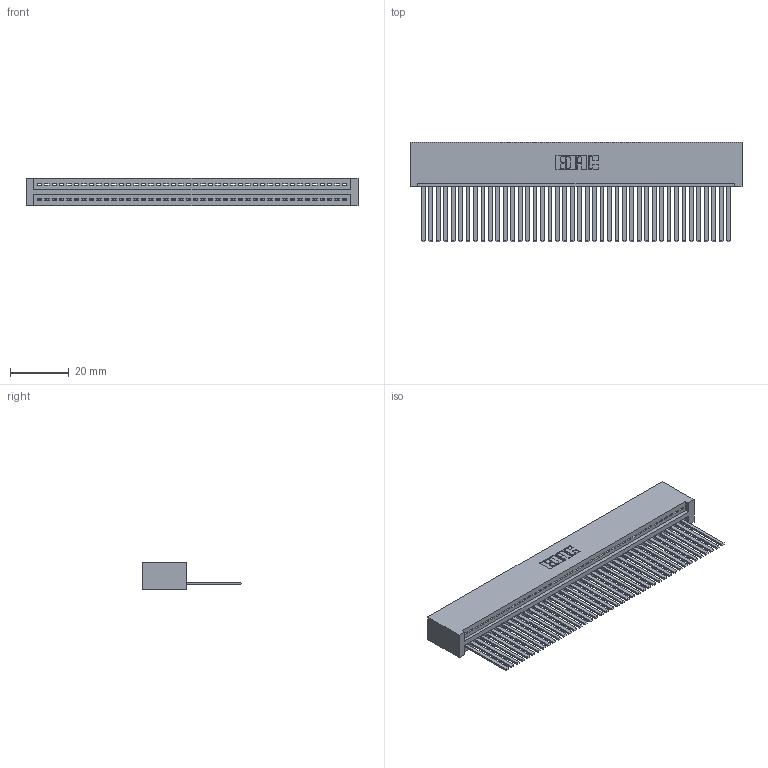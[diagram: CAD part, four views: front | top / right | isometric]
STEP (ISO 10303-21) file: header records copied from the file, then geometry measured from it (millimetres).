
FILE_DESCRIPTION (( 'STEP AP203' ), '1' );
FILE_NAME ('395-042-544-101.STEP', '2018-11-15T11:17:45', ( '' ), ( '' ), 'SwSTEP 2.0', 'SolidWorks 2016', '' );
FILE_SCHEMA (( 'CONFIG_CONTROL_DESIGN' ));
Length unit declared in the file: inch
Products named in the file (3): 395-042-544-101; 345 Part_No Mounting Lugs; 345-292-001_345-293-144
Assembly tree (43 placements, depth 2):
  395-042-544-101
    345 Part_No Mounting Lugs
    345-292-001_345-293-144  x42
Bounding box: 113.28 x 33.96 x 9.4 mm (x, y, z)
Volume: 11830.6 mm3; surface area: 17372.2 mm2
Topology: 43 solids, 43 shells, 2302 faces, 6953 edges, 4578 vertices
Faces by surface type: plane 1588, cylinder 714
Entity records: 31149 total; most frequent: CARTESIAN_POINT 5402, ORIENTED_EDGE 5378, DIRECTION 4709, EDGE_CURVE 2689, VECTOR 2401, LINE 2401, VERTEX_POINT 1790, AXIS2_PLACEMENT_3D 1154
